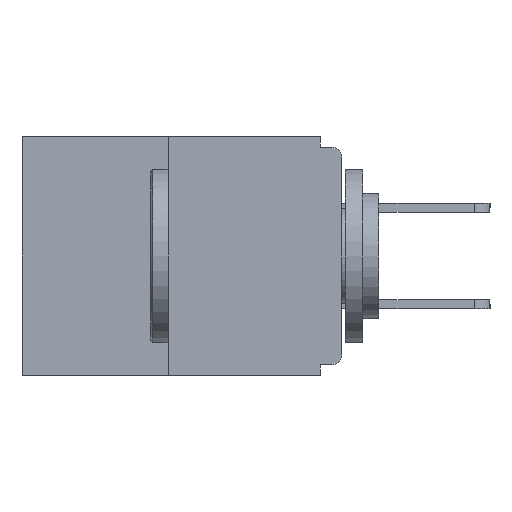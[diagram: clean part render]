
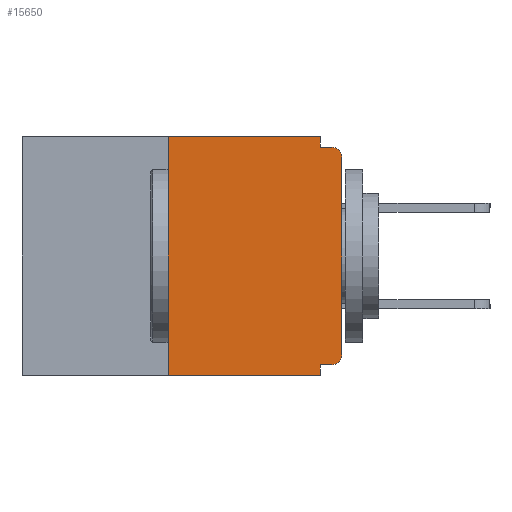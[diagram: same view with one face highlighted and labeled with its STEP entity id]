
A CAD part, left-side view. The second image highlights one B-rep face of the part: STEP entity #15650.
In plain terms, the highlighted planar face has unit normal (-1, 0, 0).
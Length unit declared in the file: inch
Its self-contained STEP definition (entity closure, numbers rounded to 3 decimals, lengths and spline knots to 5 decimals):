
#128 = DIRECTION ( 'NONE',  ( 0., -1., 0. ) ) ;
#339 = EDGE_CURVE ( 'NONE', #6358, #18377, #18095, .T. ) ;
#436 = CARTESIAN_POINT ( 'NONE',  ( 0., 0.46, 0. ) ) ;
#519 = CARTESIAN_POINT ( 'NONE',  ( 0., 0.015, -0.313 ) ) ;
#624 = ORIENTED_EDGE ( 'NONE', *, *, #2531, .F. ) ;
#1039 = VECTOR ( 'NONE', #6638, 39.37008 ) ;
#1191 = LINE ( 'NONE', #15617, #8137 ) ;
#1310 = CARTESIAN_POINT ( 'NONE',  ( 0., 0., -0.015 ) ) ;
#1634 = CARTESIAN_POINT ( 'NONE',  ( 0., 0.015, -0.328 ) ) ;
#1884 = DIRECTION ( 'NONE',  ( 0., 0., -1. ) ) ;
#2252 = VERTEX_POINT ( 'NONE', #3512 ) ;
#2343 = ORIENTED_EDGE ( 'NONE', *, *, #13278, .F. ) ;
#2437 = CARTESIAN_POINT ( 'NONE',  ( 0., 0.25, 0. ) ) ;
#2531 = EDGE_CURVE ( 'NONE', #17563, #18377, #16194, .T. ) ;
#2542 = VECTOR ( 'NONE', #3245, 39.37008 ) ;
#2585 = AXIS2_PLACEMENT_3D ( 'NONE', #519, #10537, #14896 ) ;
#2588 = CARTESIAN_POINT ( 'NONE',  ( 0., 0.015, -0.03 ) ) ;
#2614 = CARTESIAN_POINT ( 'NONE',  ( 0., 0.015, -0.015 ) ) ;
#2639 = EDGE_CURVE ( 'NONE', #5443, #6358, #1191, .T. ) ;
#2802 = EDGE_CURVE ( 'NONE', #2252, #18206, #5906, .T. ) ;
#2833 = EDGE_CURVE ( 'NONE', #6953, #2252, #15497, .T. ) ;
#3195 = DIRECTION ( 'NONE',  ( 1., 0., 0. ) ) ;
#3245 = DIRECTION ( 'NONE',  ( 0., 0., -1. ) ) ;
#3332 = FACE_OUTER_BOUND ( 'NONE', #5115, .T. ) ;
#3493 = CARTESIAN_POINT ( 'NONE',  ( 0., 0.031, -0.343 ) ) ;
#3512 = CARTESIAN_POINT ( 'NONE',  ( 0., 0.031, -0.328 ) ) ;
#4796 = ORIENTED_EDGE ( 'NONE', *, *, #5136, .T. ) ;
#5115 = EDGE_LOOP ( 'NONE', ( #8988, #17407, #4796, #10665, #13459, #7836, #7056, #16616, #624, #2343 ) ) ;
#5136 = EDGE_CURVE ( 'NONE', #9940, #18206, #16537, .T. ) ;
#5305 = LINE ( 'NONE', #16483, #15802 ) ;
#5350 = DIRECTION ( 'NONE',  ( -1., 0., 0. ) ) ;
#5443 = VERTEX_POINT ( 'NONE', #6498 ) ;
#5451 = CIRCLE ( 'NONE', #2585, 0.015 ) ;
#5906 = LINE ( 'NONE', #3493, #2542 ) ;
#5980 = DIRECTION ( 'NONE',  ( 0., 0., -1. ) ) ;
#6358 = VERTEX_POINT ( 'NONE', #6905 ) ;
#6498 = CARTESIAN_POINT ( 'NONE',  ( 0., 0., -0.313 ) ) ;
#6638 = DIRECTION ( 'NONE',  ( 0., -1., 0. ) ) ;
#6905 = CARTESIAN_POINT ( 'NONE',  ( 0., 0., -0.03 ) ) ;
#6953 = VERTEX_POINT ( 'NONE', #1634 ) ;
#7056 = ORIENTED_EDGE ( 'NONE', *, *, #2639, .T. ) ;
#7453 = VECTOR ( 'NONE', #5980, 39.37008 ) ;
#7836 = ORIENTED_EDGE ( 'NONE', *, *, #13410, .T. ) ;
#8137 = VECTOR ( 'NONE', #8384, 39.37008 ) ;
#8384 = DIRECTION ( 'NONE',  ( 0., 0., 1. ) ) ;
#8742 = EDGE_CURVE ( 'NONE', #9940, #17775, #5305, .T. ) ;
#8988 = ORIENTED_EDGE ( 'NONE', *, *, #17129, .F. ) ;
#9285 = VECTOR ( 'NONE', #10013, 39.37008 ) ;
#9536 = DIRECTION ( 'NONE',  ( 0., 0., -1. ) ) ;
#9725 = CARTESIAN_POINT ( 'NONE',  ( 0., 0.46, 0. ) ) ;
#9797 = AXIS2_PLACEMENT_3D ( 'NONE', #436, #3195, #1884 ) ;
#9940 = VERTEX_POINT ( 'NONE', #10871 ) ;
#10013 = DIRECTION ( 'NONE',  ( 0., -1., 0. ) ) ;
#10281 = VECTOR ( 'NONE', #128, 39.37008 ) ;
#10537 = DIRECTION ( 'NONE',  ( -1., 0., 0. ) ) ;
#10570 = CARTESIAN_POINT ( 'NONE',  ( 0., 0., -0.328 ) ) ;
#10601 = VECTOR ( 'NONE', #17575, 39.37008 ) ;
#10665 = ORIENTED_EDGE ( 'NONE', *, *, #2802, .F. ) ;
#10871 = CARTESIAN_POINT ( 'NONE',  ( 0., 0.25, -0.343 ) ) ;
#11366 = CARTESIAN_POINT ( 'NONE',  ( 0., 0.031, 0. ) ) ;
#11698 = CARTESIAN_POINT ( 'NONE',  ( 0., 0.46, -0.343 ) ) ;
#11701 = LINE ( 'NONE', #14526, #7453 ) ;
#11769 = CARTESIAN_POINT ( 'NONE',  ( 0., 0.031, -0.015 ) ) ;
#12128 = VERTEX_POINT ( 'NONE', #11366 ) ;
#12157 = DIRECTION ( 'NONE',  ( 0., 0., 1. ) ) ;
#13278 = EDGE_CURVE ( 'NONE', #12128, #17563, #11701, .T. ) ;
#13410 = EDGE_CURVE ( 'NONE', #6953, #5443, #5451, .T. ) ;
#13459 = ORIENTED_EDGE ( 'NONE', *, *, #2833, .F. ) ;
#13557 = AXIS2_PLACEMENT_3D ( 'NONE', #2588, #5350, #9536 ) ;
#14526 = CARTESIAN_POINT ( 'NONE',  ( 0., 0.031, 0. ) ) ;
#14572 = PLANE ( 'NONE',  #9797 ) ;
#14896 = DIRECTION ( 'NONE',  ( 0., 0., -1. ) ) ;
#15497 = LINE ( 'NONE', #10570, #10601 ) ;
#15617 = CARTESIAN_POINT ( 'NONE',  ( 0., 0., 0. ) ) ;
#15650 = ADVANCED_FACE ( 'NONE', ( #3332 ), #14572, .F. ) ;
#15802 = VECTOR ( 'NONE', #12157, 39.37008 ) ;
#16184 = CARTESIAN_POINT ( 'NONE',  ( 0., 0.031, -0.343 ) ) ;
#16194 = LINE ( 'NONE', #1310, #9285 ) ;
#16483 = CARTESIAN_POINT ( 'NONE',  ( 0., 0.25, 0. ) ) ;
#16537 = LINE ( 'NONE', #11698, #10281 ) ;
#16616 = ORIENTED_EDGE ( 'NONE', *, *, #339, .T. ) ;
#17129 = EDGE_CURVE ( 'NONE', #17775, #12128, #17166, .T. ) ;
#17166 = LINE ( 'NONE', #9725, #1039 ) ;
#17407 = ORIENTED_EDGE ( 'NONE', *, *, #8742, .F. ) ;
#17563 = VERTEX_POINT ( 'NONE', #11769 ) ;
#17575 = DIRECTION ( 'NONE',  ( 0., 1., 0. ) ) ;
#17775 = VERTEX_POINT ( 'NONE', #2437 ) ;
#18095 = CIRCLE ( 'NONE', #13557, 0.015 ) ;
#18206 = VERTEX_POINT ( 'NONE', #16184 ) ;
#18377 = VERTEX_POINT ( 'NONE', #2614 ) ;
